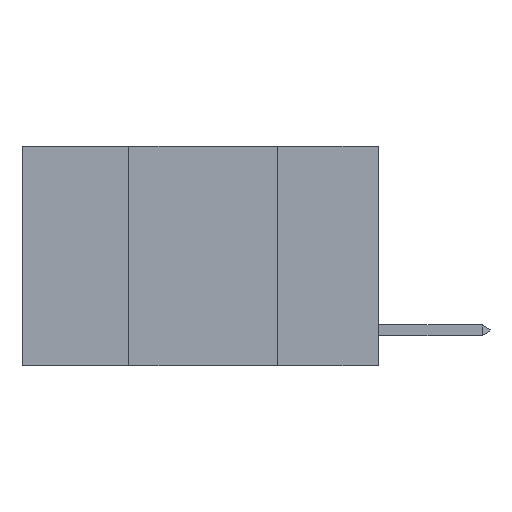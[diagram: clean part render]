
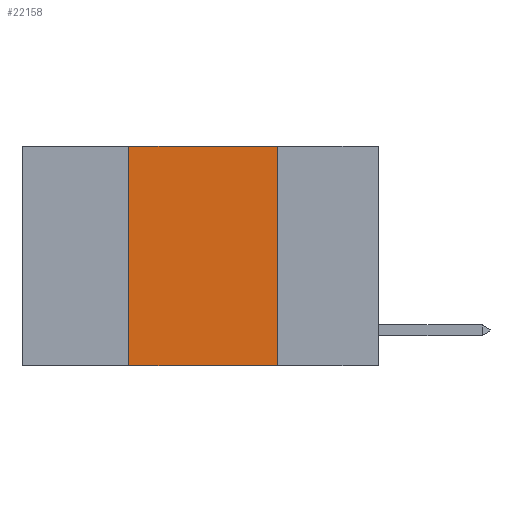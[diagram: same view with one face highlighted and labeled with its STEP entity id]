
A CAD part, left-side view. The second image highlights one B-rep face of the part: STEP entity #22158.
In plain terms, the highlighted planar face has unit normal (-1, 0, 0).
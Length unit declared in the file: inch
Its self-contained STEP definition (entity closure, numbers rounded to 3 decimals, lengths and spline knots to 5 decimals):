
#872 = AXIS2_PLACEMENT_3D ( 'NONE', #13659, #13515, #6612 ) ;
#1843 = VECTOR ( 'NONE', #5444, 39.37008 ) ;
#2477 = FACE_OUTER_BOUND ( 'NONE', #19052, .T. ) ;
#2594 = EDGE_CURVE ( 'NONE', #16172, #12723, #21937, .T. ) ;
#2728 = ORIENTED_EDGE ( 'NONE', *, *, #21548, .T. ) ;
#3882 = VECTOR ( 'NONE', #20798, 39.37008 ) ;
#4317 = ORIENTED_EDGE ( 'NONE', *, *, #8864, .F. ) ;
#5444 = DIRECTION ( 'NONE',  ( 0., 0., -1. ) ) ;
#5547 = CARTESIAN_POINT ( 'NONE',  ( 0., 0.42, -0.37 ) ) ;
#6083 = CARTESIAN_POINT ( 'NONE',  ( 0., 0.17, 0. ) ) ;
#6523 = CARTESIAN_POINT ( 'NONE',  ( 0., 0.42, 0. ) ) ;
#6597 = CARTESIAN_POINT ( 'NONE',  ( 0., 0.6, 0. ) ) ;
#6612 = DIRECTION ( 'NONE',  ( 0., 0., -1. ) ) ;
#7109 = VECTOR ( 'NONE', #20856, 39.37008 ) ;
#7686 = LINE ( 'NONE', #6523, #7109 ) ;
#8864 = EDGE_CURVE ( 'NONE', #21781, #16172, #9467, .T. ) ;
#9467 = LINE ( 'NONE', #6597, #18421 ) ;
#9726 = LINE ( 'NONE', #13656, #3882 ) ;
#10851 = CARTESIAN_POINT ( 'NONE',  ( 0., 0.17, 0. ) ) ;
#12351 = VERTEX_POINT ( 'NONE', #5547 ) ;
#12723 = VERTEX_POINT ( 'NONE', #19761 ) ;
#13427 = PLANE ( 'NONE',  #872 ) ;
#13515 = DIRECTION ( 'NONE',  ( 1., 0., 0. ) ) ;
#13656 = CARTESIAN_POINT ( 'NONE',  ( 0., 0.6, -0.37 ) ) ;
#13659 = CARTESIAN_POINT ( 'NONE',  ( 0., 0.6, 0. ) ) ;
#16172 = VERTEX_POINT ( 'NONE', #6083 ) ;
#18171 = CARTESIAN_POINT ( 'NONE',  ( 0., 0.42, 0. ) ) ;
#18248 = EDGE_CURVE ( 'NONE', #12351, #21781, #7686, .T. ) ;
#18421 = VECTOR ( 'NONE', #22518, 39.37008 ) ;
#19052 = EDGE_LOOP ( 'NONE', ( #22104, #4317, #19211, #2728 ) ) ;
#19211 = ORIENTED_EDGE ( 'NONE', *, *, #18248, .F. ) ;
#19761 = CARTESIAN_POINT ( 'NONE',  ( 0., 0.17, -0.37 ) ) ;
#20798 = DIRECTION ( 'NONE',  ( 0., -1., 0. ) ) ;
#20856 = DIRECTION ( 'NONE',  ( 0., 0., 1. ) ) ;
#21548 = EDGE_CURVE ( 'NONE', #12351, #12723, #9726, .T. ) ;
#21781 = VERTEX_POINT ( 'NONE', #18171 ) ;
#21937 = LINE ( 'NONE', #10851, #1843 ) ;
#22104 = ORIENTED_EDGE ( 'NONE', *, *, #2594, .F. ) ;
#22158 = ADVANCED_FACE ( 'NONE', ( #2477 ), #13427, .F. ) ;
#22518 = DIRECTION ( 'NONE',  ( 0., -1., 0. ) ) ;
